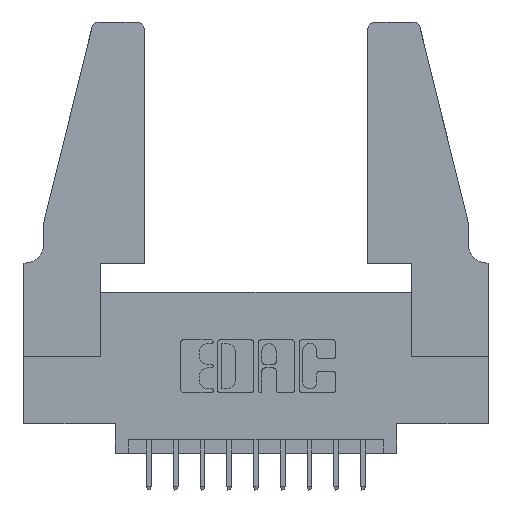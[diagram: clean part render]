
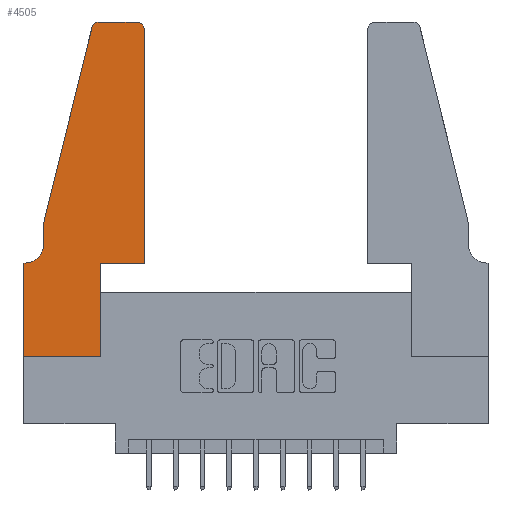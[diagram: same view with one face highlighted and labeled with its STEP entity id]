
A CAD part, top view. The second image highlights one B-rep face of the part: STEP entity #4505.
In plain terms, the highlighted planar face has unit normal (0, 0, 1).
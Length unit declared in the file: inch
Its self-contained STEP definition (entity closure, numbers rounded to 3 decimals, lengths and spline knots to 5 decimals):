
#66 = EDGE_CURVE ( 'NONE', #12604, #9186, #8002, .T. ) ;
#125 = FACE_OUTER_BOUND ( 'NONE', #9683, .T. ) ;
#167 = VERTEX_POINT ( 'NONE', #7778 ) ;
#192 = ORIENTED_EDGE ( 'NONE', *, *, #537, .T. ) ;
#319 = AXIS2_PLACEMENT_3D ( 'NONE', #3739, #12299, #7802 ) ;
#509 = CIRCLE ( 'NONE', #2295, 0.03 ) ;
#537 = EDGE_CURVE ( 'NONE', #11381, #167, #9746, .T. ) ;
#689 = VERTEX_POINT ( 'NONE', #7350 ) ;
#1099 = VECTOR ( 'NONE', #11022, 39.37008 ) ;
#1166 = DIRECTION ( 'NONE',  ( 1., 0., 0. ) ) ;
#1206 = CARTESIAN_POINT ( 'NONE',  ( 0., 0., 0.37 ) ) ;
#1271 = EDGE_CURVE ( 'NONE', #12454, #5314, #11542, .T. ) ;
#1482 = CARTESIAN_POINT ( 'NONE',  ( 0.0755, 0.42, 0.37 ) ) ;
#1703 = ORIENTED_EDGE ( 'NONE', *, *, #5374, .T. ) ;
#1898 = CARTESIAN_POINT ( 'NONE',  ( 0.0755, 0.5, 0.37 ) ) ;
#1959 = ORIENTED_EDGE ( 'NONE', *, *, #13087, .T. ) ;
#2230 = EDGE_CURVE ( 'NONE', #689, #12604, #9456, .T. ) ;
#2295 = AXIS2_PLACEMENT_3D ( 'NONE', #4545, #3416, #7824 ) ;
#2540 = CIRCLE ( 'NONE', #8576, 0.07 ) ;
#2666 = LINE ( 'NONE', #3652, #12288 ) ;
#3002 = DIRECTION ( 'NONE',  ( -1., 0., 0. ) ) ;
#3021 = CIRCLE ( 'NONE', #319, 0.03 ) ;
#3416 = DIRECTION ( 'NONE',  ( 0., 0., 1. ) ) ;
#3632 = CARTESIAN_POINT ( 'NONE',  ( 0.2865, 0.35, 0.37 ) ) ;
#3652 = CARTESIAN_POINT ( 'NONE',  ( 0.4505, 0.35, 0.37 ) ) ;
#3714 = EDGE_CURVE ( 'NONE', #9182, #5216, #509, .T. ) ;
#3739 = CARTESIAN_POINT ( 'NONE',  ( 0.4205, 1.22, 0.37 ) ) ;
#3804 = EDGE_CURVE ( 'NONE', #5314, #689, #2540, .T. ) ;
#3975 = VECTOR ( 'NONE', #5732, 39.37008 ) ;
#3999 = CARTESIAN_POINT ( 'NONE',  ( 0.2865, 0.35, 0.37 ) ) ;
#4503 = ORIENTED_EDGE ( 'NONE', *, *, #2230, .T. ) ;
#4505 = ADVANCED_FACE ( 'NONE', ( #125 ), #7634, .T. ) ;
#4545 = CARTESIAN_POINT ( 'NONE',  ( 0.284, 1.22, 0.37 ) ) ;
#4711 = DIRECTION ( 'NONE',  ( -0.239, -0.971, 0. ) ) ;
#5061 = VERTEX_POINT ( 'NONE', #9802 ) ;
#5216 = VERTEX_POINT ( 'NONE', #12392 ) ;
#5314 = VERTEX_POINT ( 'NONE', #1482 ) ;
#5363 = VERTEX_POINT ( 'NONE', #11122 ) ;
#5374 = EDGE_CURVE ( 'NONE', #7669, #5061, #3021, .T. ) ;
#5525 = CARTESIAN_POINT ( 'NONE',  ( 0.4505, 0.35, 0.37 ) ) ;
#5604 = CARTESIAN_POINT ( 'NONE',  ( 0.0755, 0.5, 0.37 ) ) ;
#5732 = DIRECTION ( 'NONE',  ( 1., 0., 0. ) ) ;
#5847 = CARTESIAN_POINT ( 'NONE',  ( 0.0055, 0.42, 0.37 ) ) ;
#5924 = EDGE_CURVE ( 'NONE', #5363, #11381, #8108, .T. ) ;
#6449 = CARTESIAN_POINT ( 'NONE',  ( 0.0755, 0.5, 0.37 ) ) ;
#6525 = CARTESIAN_POINT ( 'NONE',  ( 0.284, 1.25, 0.37 ) ) ;
#7053 = ORIENTED_EDGE ( 'NONE', *, *, #5924, .T. ) ;
#7164 = CARTESIAN_POINT ( 'NONE',  ( 0., 0.35, 0.37 ) ) ;
#7312 = ORIENTED_EDGE ( 'NONE', *, *, #3714, .T. ) ;
#7350 = CARTESIAN_POINT ( 'NONE',  ( 0.0055, 0.35, 0.37 ) ) ;
#7474 = AXIS2_PLACEMENT_3D ( 'NONE', #7164, #12579, #10800 ) ;
#7634 = PLANE ( 'NONE',  #7474 ) ;
#7669 = VERTEX_POINT ( 'NONE', #8426 ) ;
#7778 = CARTESIAN_POINT ( 'NONE',  ( 0.4505, 0.35, 0.37 ) ) ;
#7802 = DIRECTION ( 'NONE',  ( 1., 0., 0. ) ) ;
#7824 = DIRECTION ( 'NONE',  ( 1., 0., 0. ) ) ;
#7988 = DIRECTION ( 'NONE',  ( 0., 1., 0. ) ) ;
#8002 = LINE ( 'NONE', #12361, #11798 ) ;
#8108 = LINE ( 'NONE', #3632, #10204 ) ;
#8201 = DIRECTION ( 'NONE',  ( 0., -1., 0. ) ) ;
#8321 = VECTOR ( 'NONE', #8201, 39.37008 ) ;
#8338 = VECTOR ( 'NONE', #3002, 39.37008 ) ;
#8426 = CARTESIAN_POINT ( 'NONE',  ( 0.4505, 1.22, 0.37 ) ) ;
#8552 = ORIENTED_EDGE ( 'NONE', *, *, #8786, .T. ) ;
#8576 = AXIS2_PLACEMENT_3D ( 'NONE', #5847, #10217, #12321 ) ;
#8714 = VECTOR ( 'NONE', #4711, 39.37008 ) ;
#8786 = EDGE_CURVE ( 'NONE', #9186, #5363, #11006, .T. ) ;
#9101 = DIRECTION ( 'NONE',  ( 0., 1., 0. ) ) ;
#9182 = VERTEX_POINT ( 'NONE', #6525 ) ;
#9186 = VERTEX_POINT ( 'NONE', #1206 ) ;
#9456 = LINE ( 'NONE', #11778, #8338 ) ;
#9683 = EDGE_LOOP ( 'NONE', ( #1959, #7312, #11111, #11573, #11097, #4503, #13128, #8552, #7053, #192, #13592, #1703 ) ) ;
#9746 = LINE ( 'NONE', #5525, #11704 ) ;
#9802 = CARTESIAN_POINT ( 'NONE',  ( 0.4205, 1.25, 0.37 ) ) ;
#10106 = LINE ( 'NONE', #5604, #8714 ) ;
#10204 = VECTOR ( 'NONE', #9101, 39.37008 ) ;
#10217 = DIRECTION ( 'NONE',  ( 0., 0., -1. ) ) ;
#10800 = DIRECTION ( 'NONE',  ( 1., 0., 0. ) ) ;
#11006 = LINE ( 'NONE', #13441, #3975 ) ;
#11022 = DIRECTION ( 'NONE',  ( -1., 0., 0. ) ) ;
#11097 = ORIENTED_EDGE ( 'NONE', *, *, #3804, .T. ) ;
#11111 = ORIENTED_EDGE ( 'NONE', *, *, #13027, .T. ) ;
#11122 = CARTESIAN_POINT ( 'NONE',  ( 0.2865, 0., 0.37 ) ) ;
#11381 = VERTEX_POINT ( 'NONE', #3999 ) ;
#11542 = LINE ( 'NONE', #1898, #8321 ) ;
#11573 = ORIENTED_EDGE ( 'NONE', *, *, #1271, .T. ) ;
#11627 = EDGE_CURVE ( 'NONE', #167, #7669, #2666, .T. ) ;
#11704 = VECTOR ( 'NONE', #1166, 39.37008 ) ;
#11778 = CARTESIAN_POINT ( 'NONE',  ( 0.0755, 0.35, 0.37 ) ) ;
#11798 = VECTOR ( 'NONE', #13556, 39.37008 ) ;
#12288 = VECTOR ( 'NONE', #7988, 39.37008 ) ;
#12299 = DIRECTION ( 'NONE',  ( 0., 0., 1. ) ) ;
#12321 = DIRECTION ( 'NONE',  ( -1., 0., 0. ) ) ;
#12361 = CARTESIAN_POINT ( 'NONE',  ( 0., 0., 0.37 ) ) ;
#12392 = CARTESIAN_POINT ( 'NONE',  ( 0.25487, 1.22718, 0.37 ) ) ;
#12454 = VERTEX_POINT ( 'NONE', #6449 ) ;
#12579 = DIRECTION ( 'NONE',  ( 0., 0., 1. ) ) ;
#12604 = VERTEX_POINT ( 'NONE', #13418 ) ;
#13027 = EDGE_CURVE ( 'NONE', #5216, #12454, #10106, .T. ) ;
#13087 = EDGE_CURVE ( 'NONE', #5061, #9182, #13263, .T. ) ;
#13128 = ORIENTED_EDGE ( 'NONE', *, *, #66, .T. ) ;
#13263 = LINE ( 'NONE', #13332, #1099 ) ;
#13332 = CARTESIAN_POINT ( 'NONE',  ( 0.2605, 1.25, 0.37 ) ) ;
#13418 = CARTESIAN_POINT ( 'NONE',  ( 0., 0.35, 0.37 ) ) ;
#13441 = CARTESIAN_POINT ( 'NONE',  ( 0., 0., 0.37 ) ) ;
#13556 = DIRECTION ( 'NONE',  ( 0., -1., 0. ) ) ;
#13592 = ORIENTED_EDGE ( 'NONE', *, *, #11627, .T. ) ;
